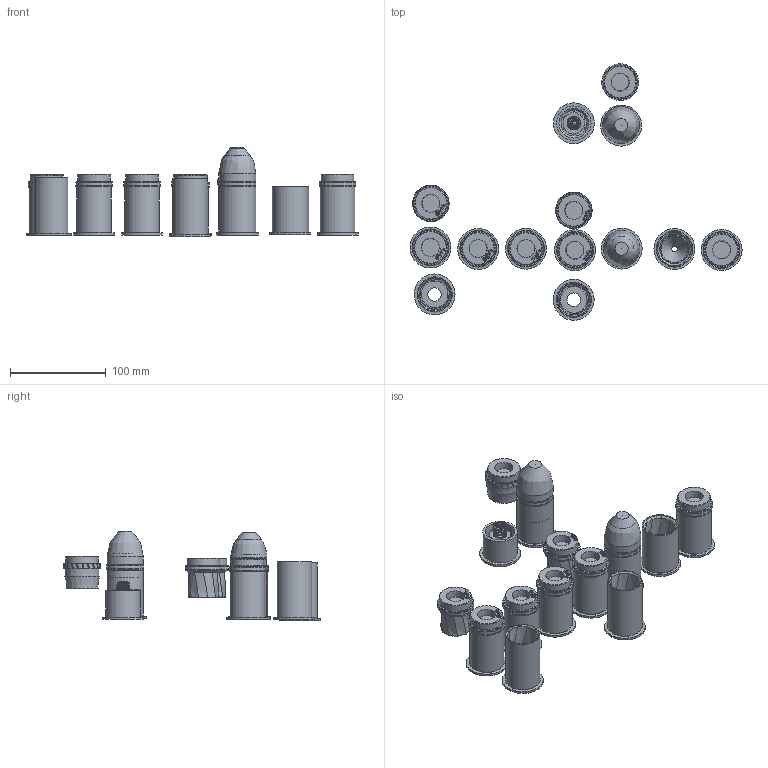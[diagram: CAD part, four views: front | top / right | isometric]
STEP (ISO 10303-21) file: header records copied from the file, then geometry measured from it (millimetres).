
FILE_DESCRIPTION(/* description */ (''),/* implementation_level */ '2;1');
FILE_NAME(/* name */ 'MILC Assembly & Projectiles.step',/* time_stamp */ '2023-01-12T07:08:48-05:00',/* author */ (''),/* organization */ (''),/* preprocessor_version */ 'ST-DEVELOPER v19.2',/* originating_system */ 'Autodesk Translation Framework v11.17.0.187',/* authorisation */ '');
FILE_SCHEMA (('AUTOMOTIVE_DESIGN { 1 0 10303 214 3 1 1 }'));
Length unit declared in the file: millimetre
Products named in the file (45): JP Rifld MILC MULTI RATE 2.5; JP Polygonal Rifled 37mm; JP Poly Rifled MILC Shell Casing; Brass Sleeve v3 (1); 209 Shell Casing; Brass Sleeve v3 (1) (2); JP Poly Rifled M781 37mm; Base Pusher (1); Windshield (1); 91310A762_High-Strength Class 10.9 Steel Hex Head Screw (1); 1:24; 1:24 Pusher; 1:24 Casing; 1:36; 1:36 Pusher; 1:36 Casing; Blank For Mods; Pusher; Casing; 1:12; 1:12 Pusher Fencepost; 1:12 Casing; 1:48; 1:48 Pusher Fencpost; 1:48 Casing; 1:12 Seamless; 1:48 Seamless; 1:48 LongMILC; 1:48 Casing_1; 1:12 LongMILC; 1:12 Casing_1; MILC M781 Full Assembly; 92015A139_18-8 Stainless Steel Cup-Point Set Screw; 90592A032_Steel Hex Nut; 91310A762_High-Strength Class 10.9 Steel Hex Head Screw; M781 37mm Rev A; Base Pusher; Windshield; Brass Sleeve; 209 MILC ...
Assembly tree (44 placements, depth 5):
  JP Rifld MILC MULTI RATE 2.5
    JP Polygonal Rifled 37mm
      JP Poly Rifled MILC Shell Casing
        Brass Sleeve v3 (1)
        209 Shell Casing
          Brass Sleeve v3 (1) (2)
      JP Poly Rifled M781 37mm
        Base Pusher (1)
        Windshield (1)
      91310A762_High-Strength Class 10.9 Steel Hex Head Screw (1)
      1:24
        1:24 Pusher
        1:24 Casing
      1:36
        1:36 Pusher
        1:36 Casing
      Blank For Mods
        Pusher
        Casing
    1:12
      1:12 Pusher Fencepost
      1:12 Casing
    1:48
      1:48 Pusher Fencpost
      1:48 Casing
    1:12 Seamless
    1:48 Seamless
    1:48 LongMILC
      1:48 Casing_1
    1:12 LongMILC
      1:12 Casing_1
    MILC M781 Full Assembly
      92015A139_18-8 Stainless Steel Cup-Point Set Screw
      90592A032_Steel Hex Nut
      91310A762_High-Strength Class 10.9 Steel Hex Head Screw
      M781 37mm Rev A
        Base Pusher
        Windshield
      Brass Sleeve
    209 MILC
      90592A032_Steel Hex Nut_1
      91310A762_High-Strength Class 10.9 Steel Hex Head Screw_1
      92311A615_18-8 Stainless Steel Cup-Point Set Screw
    M781 Rifled Pusher
      Base Pusher_1
Bounding box: 347.38 x 268.28 x 93.75 mm (x, y, z)
Volume: 545145.6 mm3; surface area: 277312.8 mm2
Topology: 33 solids, 33 shells, 2455 faces, 6383 edges, 4174 vertices
Faces by surface type: bspline 1273, plane 702, cylinder 291, cone 146, torus 43
Full cylindrical faces by diameter (mm): 3 x12, 6.195 x1, 6.376 x5, 6.779 x3, 7.463 x3, 7.94 x2, 8 x5, 9.525 x1, 9.85 x2, 11.2 x2, 11.402 x45, 14 x46, 14.2 x10, 28 x8, 31 x2, 34 x12, 36.1 x11, 36.2 x3, 37.6 x2, 38 x9, 38.123 x2, 38.188 x1, 38.3 x2, 38.5 x7, 42.8 x11
Entity records: 188976 total; most frequent: CARTESIAN_POINT 136658, ORIENTED_EDGE 12750, DIRECTION 6808, EDGE_CURVE 6375, VERTEX_POINT 4173, EDGE_LOOP 2704, LINE 2692, VECTOR 2692
